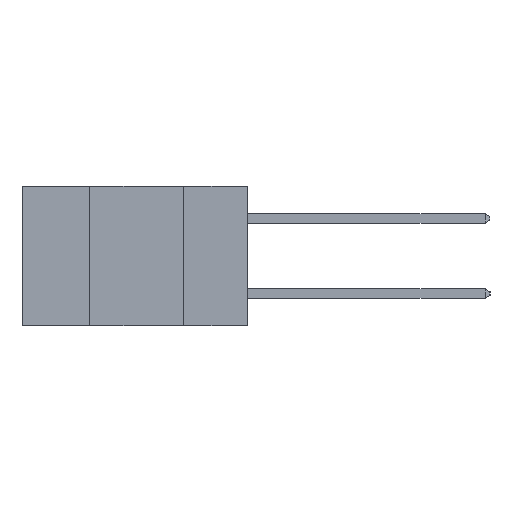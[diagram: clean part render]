
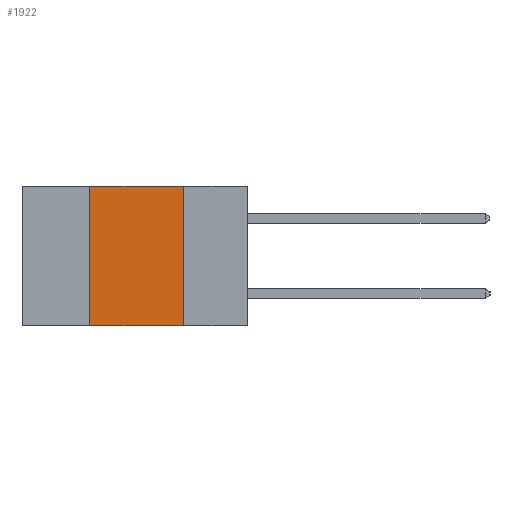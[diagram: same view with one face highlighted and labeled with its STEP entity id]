
A CAD part, left-side view. The second image highlights one B-rep face of the part: STEP entity #1922.
In plain terms, the highlighted planar face has unit normal (-1, 0, 0).
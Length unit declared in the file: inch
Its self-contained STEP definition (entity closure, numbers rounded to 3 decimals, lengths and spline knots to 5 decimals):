
#253 = DIRECTION ( 'NONE',  ( 0., -1., 0. ) ) ;
#364 = ORIENTED_EDGE ( 'NONE', *, *, #1127, .T. ) ;
#723 = CARTESIAN_POINT ( 'NONE',  ( 0., 0.6, 0. ) ) ;
#749 = LINE ( 'NONE', #723, #8866 ) ;
#855 = EDGE_CURVE ( 'NONE', #1325, #8420, #8361, .T. ) ;
#1127 = EDGE_CURVE ( 'NONE', #1325, #8622, #11278, .T. ) ;
#1325 = VERTEX_POINT ( 'NONE', #8598 ) ;
#1359 = AXIS2_PLACEMENT_3D ( 'NONE', #13794, #9276, #9272 ) ;
#1922 = ADVANCED_FACE ( 'NONE', ( #12197 ), #10405, .F. ) ;
#2444 = VECTOR ( 'NONE', #5355, 39.37008 ) ;
#2478 = VECTOR ( 'NONE', #12587, 39.37008 ) ;
#2694 = EDGE_CURVE ( 'NONE', #10430, #8622, #5097, .T. ) ;
#5081 = CARTESIAN_POINT ( 'NONE',  ( 0., 0.42, -0.37 ) ) ;
#5097 = LINE ( 'NONE', #12022, #2478 ) ;
#5355 = DIRECTION ( 'NONE',  ( 0., 0., 1. ) ) ;
#5482 = CARTESIAN_POINT ( 'NONE',  ( 0., 0.17, -0.37 ) ) ;
#5885 = CARTESIAN_POINT ( 'NONE',  ( 0., 0.17, 0. ) ) ;
#5944 = ORIENTED_EDGE ( 'NONE', *, *, #9737, .F. ) ;
#8241 = DIRECTION ( 'NONE',  ( 0., -1., 0. ) ) ;
#8360 = CARTESIAN_POINT ( 'NONE',  ( 0., 0.6, -0.37 ) ) ;
#8361 = LINE ( 'NONE', #5081, #2444 ) ;
#8420 = VERTEX_POINT ( 'NONE', #8628 ) ;
#8503 = ORIENTED_EDGE ( 'NONE', *, *, #2694, .F. ) ;
#8598 = CARTESIAN_POINT ( 'NONE',  ( 0., 0.42, -0.37 ) ) ;
#8622 = VERTEX_POINT ( 'NONE', #5482 ) ;
#8628 = CARTESIAN_POINT ( 'NONE',  ( 0., 0.42, 0. ) ) ;
#8818 = ORIENTED_EDGE ( 'NONE', *, *, #855, .F. ) ;
#8866 = VECTOR ( 'NONE', #253, 39.37008 ) ;
#9272 = DIRECTION ( 'NONE',  ( 0., 0., -1. ) ) ;
#9276 = DIRECTION ( 'NONE',  ( 1., 0., 0. ) ) ;
#9737 = EDGE_CURVE ( 'NONE', #8420, #10430, #749, .T. ) ;
#10405 = PLANE ( 'NONE',  #1359 ) ;
#10430 = VERTEX_POINT ( 'NONE', #5885 ) ;
#11278 = LINE ( 'NONE', #8360, #13284 ) ;
#12022 = CARTESIAN_POINT ( 'NONE',  ( 0., 0.17, -0.37 ) ) ;
#12197 = FACE_OUTER_BOUND ( 'NONE', #12729, .T. ) ;
#12587 = DIRECTION ( 'NONE',  ( 0., 0., -1. ) ) ;
#12729 = EDGE_LOOP ( 'NONE', ( #8503, #5944, #8818, #364 ) ) ;
#13284 = VECTOR ( 'NONE', #8241, 39.37008 ) ;
#13794 = CARTESIAN_POINT ( 'NONE',  ( 0., 0.6, 0. ) ) ;
